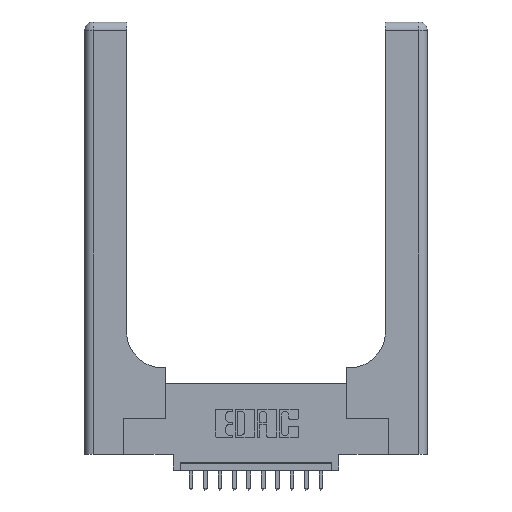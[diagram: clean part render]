
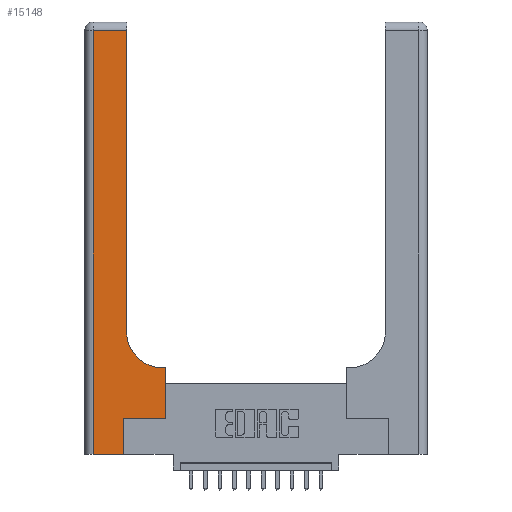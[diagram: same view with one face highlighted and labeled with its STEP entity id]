
A CAD part, top view. The second image highlights one B-rep face of the part: STEP entity #15148.
In plain terms, the highlighted planar face has unit normal (0, 0, 1).
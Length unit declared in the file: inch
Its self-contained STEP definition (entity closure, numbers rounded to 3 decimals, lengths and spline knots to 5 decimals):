
#46 = CARTESIAN_POINT ( 'NONE',  ( 0.269, 0.25, 0.37 ) ) ;
#218 = EDGE_CURVE ( 'NONE', #4519, #10894, #6071, .T. ) ;
#243 = ORIENTED_EDGE ( 'NONE', *, *, #2704, .T. ) ;
#248 = PLANE ( 'NONE',  #10132 ) ;
#303 = CARTESIAN_POINT ( 'NONE',  ( 0., 3., 0.37 ) ) ;
#673 = ORIENTED_EDGE ( 'NONE', *, *, #7316, .T. ) ;
#1285 = VERTEX_POINT ( 'NONE', #4721 ) ;
#1447 = CARTESIAN_POINT ( 'NONE',  ( 0., 0., 0.37 ) ) ;
#1773 = DIRECTION ( 'NONE',  ( 1., 0., 0. ) ) ;
#2110 = VECTOR ( 'NONE', #9689, 39.37008 ) ;
#2407 = DIRECTION ( 'NONE',  ( -1., 0., 0. ) ) ;
#2704 = EDGE_CURVE ( 'NONE', #8236, #1285, #11807, .T. ) ;
#2888 = ORIENTED_EDGE ( 'NONE', *, *, #12727, .T. ) ;
#3055 = CARTESIAN_POINT ( 'NONE',  ( 0.2915, 2.94, 0.37 ) ) ;
#3156 = DIRECTION ( 'NONE',  ( 0., 1., 0. ) ) ;
#3487 = VECTOR ( 'NONE', #2407, 39.37008 ) ;
#3846 = AXIS2_PLACEMENT_3D ( 'NONE', #16462, #11053, #1773 ) ;
#3968 = DIRECTION ( 'NONE',  ( 1., 0., 0. ) ) ;
#3980 = DIRECTION ( 'NONE',  ( 0., 1., 0. ) ) ;
#4030 = CARTESIAN_POINT ( 'NONE',  ( 0.06, 0., 0.37 ) ) ;
#4289 = CARTESIAN_POINT ( 'NONE',  ( 0.06, 3., 0.37 ) ) ;
#4343 = VECTOR ( 'NONE', #3156, 39.37008 ) ;
#4352 = VERTEX_POINT ( 'NONE', #17006 ) ;
#4519 = VERTEX_POINT ( 'NONE', #11180 ) ;
#4721 = CARTESIAN_POINT ( 'NONE',  ( 0.5585, 0.6, 0.37 ) ) ;
#4760 = VERTEX_POINT ( 'NONE', #3055 ) ;
#4877 = EDGE_LOOP ( 'NONE', ( #9254, #2888, #12854, #673, #15617, #9649, #243, #14458, #10576 ) ) ;
#5163 = EDGE_CURVE ( 'NONE', #6781, #8236, #10051, .T. ) ;
#5305 = VECTOR ( 'NONE', #11905, 39.37008 ) ;
#5562 = EDGE_CURVE ( 'NONE', #12960, #4352, #6548, .T. ) ;
#5581 = LINE ( 'NONE', #11914, #12229 ) ;
#6071 = LINE ( 'NONE', #4289, #2110 ) ;
#6447 = CARTESIAN_POINT ( 'NONE',  ( 0.2915, 0.6, 0.37 ) ) ;
#6548 = CIRCLE ( 'NONE', #3846, 0.25 ) ;
#6592 = LINE ( 'NONE', #16909, #3487 ) ;
#6621 = CARTESIAN_POINT ( 'NONE',  ( 0.269, 0.25, 0.37 ) ) ;
#6781 = VERTEX_POINT ( 'NONE', #46 ) ;
#6922 = CARTESIAN_POINT ( 'NONE',  ( 0.5585, 0.25, 0.37 ) ) ;
#7058 = EDGE_CURVE ( 'NONE', #1285, #12960, #8612, .T. ) ;
#7316 = EDGE_CURVE ( 'NONE', #10894, #12220, #15228, .T. ) ;
#8110 = DIRECTION ( 'NONE',  ( 1., 0., 0. ) ) ;
#8236 = VERTEX_POINT ( 'NONE', #10823 ) ;
#8382 = DIRECTION ( 'NONE',  ( 0., 0., -1. ) ) ;
#8471 = CARTESIAN_POINT ( 'NONE',  ( 0.2915, 3., 0.37 ) ) ;
#8593 = VECTOR ( 'NONE', #8110, 39.37008 ) ;
#8612 = LINE ( 'NONE', #6447, #5305 ) ;
#9074 = FACE_OUTER_BOUND ( 'NONE', #4877, .T. ) ;
#9254 = ORIENTED_EDGE ( 'NONE', *, *, #14032, .T. ) ;
#9625 = DIRECTION ( 'NONE',  ( -1., 0., 0. ) ) ;
#9649 = ORIENTED_EDGE ( 'NONE', *, *, #5163, .T. ) ;
#9689 = DIRECTION ( 'NONE',  ( 0., -1., 0. ) ) ;
#9854 = VECTOR ( 'NONE', #3968, 39.37008 ) ;
#10051 = LINE ( 'NONE', #6621, #9854 ) ;
#10132 = AXIS2_PLACEMENT_3D ( 'NONE', #303, #8382, #9625 ) ;
#10576 = ORIENTED_EDGE ( 'NONE', *, *, #5562, .T. ) ;
#10823 = CARTESIAN_POINT ( 'NONE',  ( 0.5585, 0.25, 0.37 ) ) ;
#10868 = CARTESIAN_POINT ( 'NONE',  ( 0.269, 0., 0.37 ) ) ;
#10894 = VERTEX_POINT ( 'NONE', #4030 ) ;
#11053 = DIRECTION ( 'NONE',  ( 0., 0., -1. ) ) ;
#11131 = DIRECTION ( 'NONE',  ( 0., 1., 0. ) ) ;
#11175 = LINE ( 'NONE', #8471, #15719 ) ;
#11180 = CARTESIAN_POINT ( 'NONE',  ( 0.06, 2.94, 0.37 ) ) ;
#11499 = CARTESIAN_POINT ( 'NONE',  ( 0.5415, 0.6, 0.37 ) ) ;
#11807 = LINE ( 'NONE', #6922, #4343 ) ;
#11905 = DIRECTION ( 'NONE',  ( -1., 0., 0. ) ) ;
#11914 = CARTESIAN_POINT ( 'NONE',  ( 0.269, 0., 0.37 ) ) ;
#11957 = EDGE_CURVE ( 'NONE', #12220, #6781, #5581, .T. ) ;
#12220 = VERTEX_POINT ( 'NONE', #10868 ) ;
#12229 = VECTOR ( 'NONE', #3980, 39.37008 ) ;
#12727 = EDGE_CURVE ( 'NONE', #4760, #4519, #6592, .T. ) ;
#12854 = ORIENTED_EDGE ( 'NONE', *, *, #218, .T. ) ;
#12960 = VERTEX_POINT ( 'NONE', #11499 ) ;
#14032 = EDGE_CURVE ( 'NONE', #4352, #4760, #11175, .T. ) ;
#14458 = ORIENTED_EDGE ( 'NONE', *, *, #7058, .T. ) ;
#15148 = ADVANCED_FACE ( 'NONE', ( #9074 ), #248, .F. ) ;
#15228 = LINE ( 'NONE', #1447, #8593 ) ;
#15617 = ORIENTED_EDGE ( 'NONE', *, *, #11957, .T. ) ;
#15719 = VECTOR ( 'NONE', #11131, 39.37008 ) ;
#16462 = CARTESIAN_POINT ( 'NONE',  ( 0.5415, 0.85, 0.37 ) ) ;
#16909 = CARTESIAN_POINT ( 'NONE',  ( 0., 2.94, 0.37 ) ) ;
#17006 = CARTESIAN_POINT ( 'NONE',  ( 0.2915, 0.85, 0.37 ) ) ;
